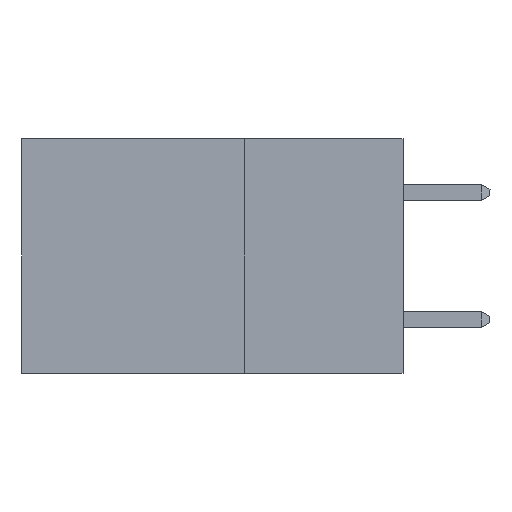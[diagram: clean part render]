
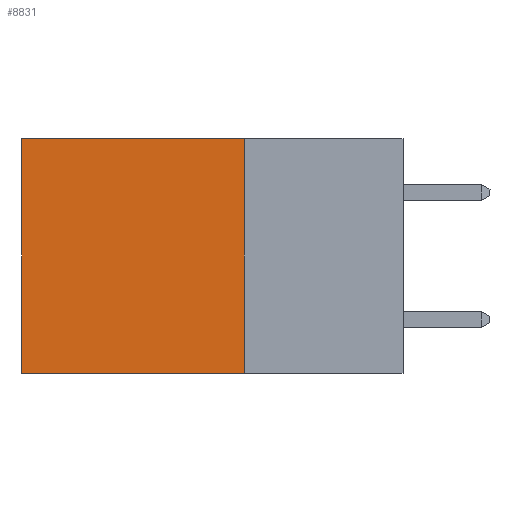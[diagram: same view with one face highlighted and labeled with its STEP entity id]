
A CAD part, left-side view. The second image highlights one B-rep face of the part: STEP entity #8831.
In plain terms, the highlighted planar face has unit normal (-1, 0, 0).
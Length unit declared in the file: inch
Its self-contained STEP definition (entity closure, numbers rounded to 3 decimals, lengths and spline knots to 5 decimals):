
#600 = CARTESIAN_POINT ( 'NONE',  ( 0.2875, 0.25, -0.37 ) ) ;
#768 = DIRECTION ( 'NONE',  ( 1., 0., 0. ) ) ;
#1304 = VECTOR ( 'NONE', #8988, 39.37008 ) ;
#1411 = ORIENTED_EDGE ( 'NONE', *, *, #3405, .F. ) ;
#1810 = LINE ( 'NONE', #5100, #6632 ) ;
#1845 = LINE ( 'NONE', #7771, #2952 ) ;
#1931 = CARTESIAN_POINT ( 'NONE',  ( 0.2875, 0.6, -0.37 ) ) ;
#2179 = VECTOR ( 'NONE', #4787, 39.37008 ) ;
#2952 = VECTOR ( 'NONE', #8855, 39.37008 ) ;
#3316 = CARTESIAN_POINT ( 'NONE',  ( 0.2875, 0.25, 0. ) ) ;
#3405 = EDGE_CURVE ( 'NONE', #5114, #8582, #4828, .T. ) ;
#3849 = FACE_OUTER_BOUND ( 'NONE', #8200, .T. ) ;
#4056 = DIRECTION ( 'NONE',  ( 0., 0., -1. ) ) ;
#4787 = DIRECTION ( 'NONE',  ( 0., 1., 0. ) ) ;
#4828 = LINE ( 'NONE', #8505, #2179 ) ;
#5100 = CARTESIAN_POINT ( 'NONE',  ( 0.2875, 0.6, 0. ) ) ;
#5114 = VERTEX_POINT ( 'NONE', #600 ) ;
#5310 = CARTESIAN_POINT ( 'NONE',  ( 0.2875, 0.6, 0. ) ) ;
#5900 = PLANE ( 'NONE',  #7510 ) ;
#6027 = CARTESIAN_POINT ( 'NONE',  ( 0.2875, 0.25, 0. ) ) ;
#6463 = ORIENTED_EDGE ( 'NONE', *, *, #7850, .F. ) ;
#6632 = VECTOR ( 'NONE', #4056, 39.37008 ) ;
#7510 = AXIS2_PLACEMENT_3D ( 'NONE', #10621, #768, #7949 ) ;
#7771 = CARTESIAN_POINT ( 'NONE',  ( 0.2875, 0.25, 0. ) ) ;
#7834 = ORIENTED_EDGE ( 'NONE', *, *, #9911, .T. ) ;
#7843 = ORIENTED_EDGE ( 'NONE', *, *, #8723, .T. ) ;
#7850 = EDGE_CURVE ( 'NONE', #12015, #5114, #1845, .T. ) ;
#7949 = DIRECTION ( 'NONE',  ( 0., 0., -1. ) ) ;
#8200 = EDGE_LOOP ( 'NONE', ( #7843, #1411, #6463, #7834 ) ) ;
#8505 = CARTESIAN_POINT ( 'NONE',  ( 0.2875, 0.25, -0.37 ) ) ;
#8582 = VERTEX_POINT ( 'NONE', #1931 ) ;
#8723 = EDGE_CURVE ( 'NONE', #9371, #8582, #1810, .T. ) ;
#8831 = ADVANCED_FACE ( 'NONE', ( #3849 ), #5900, .F. ) ;
#8855 = DIRECTION ( 'NONE',  ( 0., 0., -1. ) ) ;
#8988 = DIRECTION ( 'NONE',  ( 0., 1., 0. ) ) ;
#9341 = LINE ( 'NONE', #6027, #1304 ) ;
#9371 = VERTEX_POINT ( 'NONE', #5310 ) ;
#9911 = EDGE_CURVE ( 'NONE', #12015, #9371, #9341, .T. ) ;
#10621 = CARTESIAN_POINT ( 'NONE',  ( 0.2875, 0.25, 0. ) ) ;
#12015 = VERTEX_POINT ( 'NONE', #3316 ) ;
